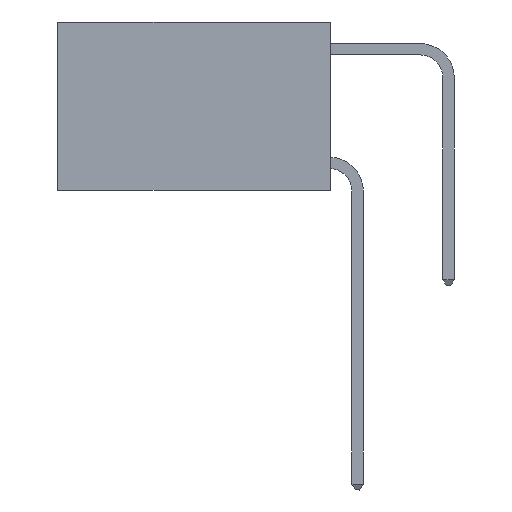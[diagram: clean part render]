
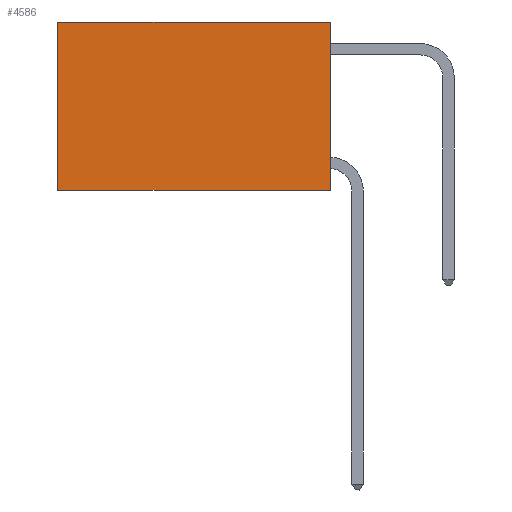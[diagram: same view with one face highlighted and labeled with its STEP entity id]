
A CAD part, left-side view. The second image highlights one B-rep face of the part: STEP entity #4586.
In plain terms, the highlighted planar face has unit normal (-1, 0, 0).
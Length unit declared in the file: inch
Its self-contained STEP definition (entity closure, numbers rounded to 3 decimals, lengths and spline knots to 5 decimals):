
#1034 = DIRECTION ( 'NONE',  ( 0., 0., -1. ) ) ;
#2921 = CARTESIAN_POINT ( 'NONE',  ( 0.2625, 0., 0. ) ) ;
#2998 = EDGE_CURVE ( 'NONE', #12982, #13062, #14914, .T. ) ;
#3973 = VECTOR ( 'NONE', #28961, 39.37008 ) ;
#4586 = ADVANCED_FACE ( 'NONE', ( #15623 ), #31413, .F. ) ;
#4678 = DIRECTION ( 'NONE',  ( 0., 0., -1. ) ) ;
#9459 = EDGE_LOOP ( 'NONE', ( #28346, #23338, #15117, #27477 ) ) ;
#12982 = VERTEX_POINT ( 'NONE', #25733 ) ;
#13062 = VERTEX_POINT ( 'NONE', #28383 ) ;
#13373 = VECTOR ( 'NONE', #1034, 39.37008 ) ;
#14012 = VERTEX_POINT ( 'NONE', #26936 ) ;
#14310 = LINE ( 'NONE', #22895, #26409 ) ;
#14388 = LINE ( 'NONE', #2921, #19299 ) ;
#14914 = LINE ( 'NONE', #30116, #13373 ) ;
#15117 = ORIENTED_EDGE ( 'NONE', *, *, #22554, .F. ) ;
#15623 = FACE_OUTER_BOUND ( 'NONE', #9459, .T. ) ;
#16906 = CARTESIAN_POINT ( 'NONE',  ( 0.2625, 0., 0. ) ) ;
#19299 = VECTOR ( 'NONE', #20083, 39.37008 ) ;
#19303 = DIRECTION ( 'NONE',  ( 1., 0., 0. ) ) ;
#20083 = DIRECTION ( 'NONE',  ( 0., 0., -1. ) ) ;
#22554 = EDGE_CURVE ( 'NONE', #14012, #24104, #14388, .T. ) ;
#22882 = AXIS2_PLACEMENT_3D ( 'NONE', #16906, #19303, #4678 ) ;
#22895 = CARTESIAN_POINT ( 'NONE',  ( 0.2625, 0., 0. ) ) ;
#23338 = ORIENTED_EDGE ( 'NONE', *, *, #23583, .F. ) ;
#23583 = EDGE_CURVE ( 'NONE', #24104, #13062, #29866, .T. ) ;
#23728 = CARTESIAN_POINT ( 'NONE',  ( 0.2625, 0., -0.37 ) ) ;
#23895 = EDGE_CURVE ( 'NONE', #14012, #12982, #14310, .T. ) ;
#24104 = VERTEX_POINT ( 'NONE', #23728 ) ;
#25321 = DIRECTION ( 'NONE',  ( 0., 1., 0. ) ) ;
#25733 = CARTESIAN_POINT ( 'NONE',  ( 0.2625, 0.6, 0. ) ) ;
#26409 = VECTOR ( 'NONE', #25321, 39.37008 ) ;
#26936 = CARTESIAN_POINT ( 'NONE',  ( 0.2625, 0., 0. ) ) ;
#27477 = ORIENTED_EDGE ( 'NONE', *, *, #23895, .T. ) ;
#28346 = ORIENTED_EDGE ( 'NONE', *, *, #2998, .T. ) ;
#28383 = CARTESIAN_POINT ( 'NONE',  ( 0.2625, 0.6, -0.37 ) ) ;
#28961 = DIRECTION ( 'NONE',  ( 0., 1., 0. ) ) ;
#29866 = LINE ( 'NONE', #31416, #3973 ) ;
#30116 = CARTESIAN_POINT ( 'NONE',  ( 0.2625, 0.6, 0. ) ) ;
#31413 = PLANE ( 'NONE',  #22882 ) ;
#31416 = CARTESIAN_POINT ( 'NONE',  ( 0.2625, 0., -0.37 ) ) ;
